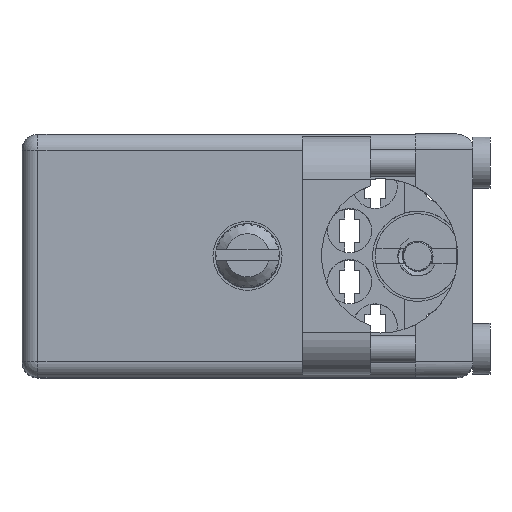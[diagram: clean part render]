
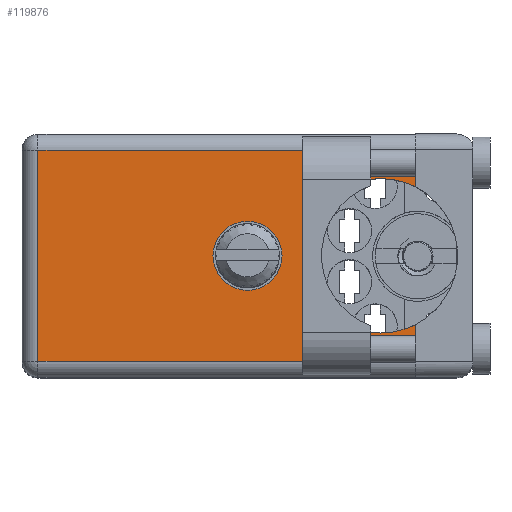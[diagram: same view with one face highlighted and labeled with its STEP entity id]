
A CAD part, top view. The second image highlights one B-rep face of the part: STEP entity #119876.
In plain terms, the highlighted face is planar.
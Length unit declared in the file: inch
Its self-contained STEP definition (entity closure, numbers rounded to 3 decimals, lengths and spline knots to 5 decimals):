
#12 = ORIENTED_EDGE ( 'NONE', *, *, #181974, .F. ) ;
#953 = EDGE_LOOP ( 'NONE', ( #184170, #178870, #45700, #61949, #62573, #991, #3942, #164983 ) ) ;
#991 = ORIENTED_EDGE ( 'NONE', *, *, #170687, .F. ) ;
#3942 = ORIENTED_EDGE ( 'NONE', *, *, #40026, .F. ) ;
#6084 = LINE ( 'NONE', #177541, #95684 ) ;
#7686 = CARTESIAN_POINT ( 'NONE',  ( 1.155, 0.906, -0.047 ) ) ;
#15477 = VERTEX_POINT ( 'NONE', #7686 ) ;
#15964 = EDGE_CURVE ( 'NONE', #175956, #15477, #23277, .T. ) ;
#17097 = EDGE_CURVE ( 'NONE', #26649, #60607, #51531, .T. ) ;
#17953 = DIRECTION ( 'NONE',  ( 0., 0., 1. ) ) ;
#20714 = AXIS2_PLACEMENT_3D ( 'NONE', #136586, #75239, #121382 ) ;
#21049 = CARTESIAN_POINT ( 'NONE',  ( 1.155, 0.906, -0.15471 ) ) ;
#22988 = CARTESIAN_POINT ( 'NONE',  ( 0.6625, 0.906, -0.3575 ) ) ;
#23277 = LINE ( 'NONE', #110480, #178972 ) ;
#26649 = VERTEX_POINT ( 'NONE', #158919 ) ;
#26757 = CARTESIAN_POINT ( 'NONE',  ( 1.155, 0.906, 0. ) ) ;
#27694 = DIRECTION ( 'NONE',  ( 0., 1., 0. ) ) ;
#28129 = CARTESIAN_POINT ( 'NONE',  ( 0.047, 0.906, -0.047 ) ) ;
#31699 = AXIS2_PLACEMENT_3D ( 'NONE', #116011, #189311, #38981 ) ;
#33539 = ORIENTED_EDGE ( 'NONE', *, *, #17097, .F. ) ;
#37393 = DIRECTION ( 'NONE',  ( 0., 1., 0. ) ) ;
#38981 = DIRECTION ( 'NONE',  ( 0., 0., 1. ) ) ;
#39547 = CIRCLE ( 'NONE', #159974, 0.227 ) ;
#39955 = DIRECTION ( 'NONE',  ( 0., 0., 1. ) ) ;
#40026 = EDGE_CURVE ( 'NONE', #125708, #55909, #39547, .T. ) ;
#45034 = VERTEX_POINT ( 'NONE', #101981 ) ;
#45109 = FACE_OUTER_BOUND ( 'NONE', #953, .T. ) ;
#45700 = ORIENTED_EDGE ( 'NONE', *, *, #111806, .T. ) ;
#51531 = CIRCLE ( 'NONE', #166721, 0.1015 ) ;
#55909 = VERTEX_POINT ( 'NONE', #116212 ) ;
#60607 = VERTEX_POINT ( 'NONE', #114581 ) ;
#61949 = ORIENTED_EDGE ( 'NONE', *, *, #15964, .T. ) ;
#62573 = ORIENTED_EDGE ( 'NONE', *, *, #193904, .F. ) ;
#62931 = VERTEX_POINT ( 'NONE', #87518 ) ;
#65061 = DIRECTION ( 'NONE',  ( 1., 0., 0. ) ) ;
#71324 = CARTESIAN_POINT ( 'NONE',  ( 1.155, 0.906, 0. ) ) ;
#72088 = DIRECTION ( 'NONE',  ( -1., 0., 0. ) ) ;
#75239 = DIRECTION ( 'NONE',  ( 0., 1., 0. ) ) ;
#83783 = EDGE_CURVE ( 'NONE', #62931, #188450, #99415, .T. ) ;
#84217 = DIRECTION ( 'NONE',  ( 0., 0., 1. ) ) ;
#87134 = DIRECTION ( 'NONE',  ( 0., 0., 1. ) ) ;
#87518 = CARTESIAN_POINT ( 'NONE',  ( 1.155, 0.906, -0.668 ) ) ;
#89527 = VERTEX_POINT ( 'NONE', #21049 ) ;
#89919 = VECTOR ( 'NONE', #39955, 39.37008 ) ;
#92616 = VECTOR ( 'NONE', #87134, 39.37008 ) ;
#95684 = VECTOR ( 'NONE', #178829, 39.37008 ) ;
#99415 = LINE ( 'NONE', #26757, #89919 ) ;
#101642 = EDGE_CURVE ( 'NONE', #188450, #125708, #107735, .T. ) ;
#101981 = CARTESIAN_POINT ( 'NONE',  ( 0.047, 0.906, -0.668 ) ) ;
#107735 = CIRCLE ( 'NONE', #31699, 0.227 ) ;
#110480 = CARTESIAN_POINT ( 'NONE',  ( 1.155, 0.906, -0.047 ) ) ;
#111565 = VECTOR ( 'NONE', #72088, 39.37008 ) ;
#111806 = EDGE_CURVE ( 'NONE', #45034, #175956, #6084, .T. ) ;
#113498 = FACE_BOUND ( 'NONE', #128687, .T. ) ;
#114581 = CARTESIAN_POINT ( 'NONE',  ( 0.6625, 0.906, -0.459 ) ) ;
#115311 = DIRECTION ( 'NONE',  ( 0., 0., 1. ) ) ;
#116011 = CARTESIAN_POINT ( 'NONE',  ( 1.053, 0.906, -0.3575 ) ) ;
#116212 = CARTESIAN_POINT ( 'NONE',  ( 1.053, 0.906, -0.1305 ) ) ;
#116341 = LINE ( 'NONE', #118855, #111565 ) ;
#118855 = CARTESIAN_POINT ( 'NONE',  ( 0., 0.906, -0.668 ) ) ;
#119876 = ADVANCED_FACE ( 'NONE', ( #45109, #113498 ), #165583, .T. ) ;
#121382 = DIRECTION ( 'NONE',  ( 0., 0., 1. ) ) ;
#123709 = AXIS2_PLACEMENT_3D ( 'NONE', #22988, #128479, #84217 ) ;
#125708 = VERTEX_POINT ( 'NONE', #181642 ) ;
#127070 = DIRECTION ( 'NONE',  ( 0., 0., 1. ) ) ;
#128479 = DIRECTION ( 'NONE',  ( 0., 1., 0. ) ) ;
#128687 = EDGE_LOOP ( 'NONE', ( #33539, #12 ) ) ;
#130353 = EDGE_CURVE ( 'NONE', #62931, #45034, #116341, .T. ) ;
#130623 = AXIS2_PLACEMENT_3D ( 'NONE', #193172, #27694, #115311 ) ;
#136586 = CARTESIAN_POINT ( 'NONE',  ( 0., 0.906, -0.715 ) ) ;
#136610 = DIRECTION ( 'NONE',  ( 0., 1., 0. ) ) ;
#141553 = CARTESIAN_POINT ( 'NONE',  ( 0.6625, 0.906, -0.3575 ) ) ;
#156234 = CARTESIAN_POINT ( 'NONE',  ( 1.155, 0.906, -0.56029 ) ) ;
#158919 = CARTESIAN_POINT ( 'NONE',  ( 0.6625, 0.906, -0.256 ) ) ;
#159974 = AXIS2_PLACEMENT_3D ( 'NONE', #168223, #136610, #17953 ) ;
#164983 = ORIENTED_EDGE ( 'NONE', *, *, #101642, .F. ) ;
#165583 = PLANE ( 'NONE',  #20714 ) ;
#165918 = LINE ( 'NONE', #71324, #92616 ) ;
#166721 = AXIS2_PLACEMENT_3D ( 'NONE', #141553, #37393, #127070 ) ;
#168223 = CARTESIAN_POINT ( 'NONE',  ( 1.053, 0.906, -0.3575 ) ) ;
#170687 = EDGE_CURVE ( 'NONE', #55909, #89527, #173046, .T. ) ;
#173046 = CIRCLE ( 'NONE', #130623, 0.227 ) ;
#175956 = VERTEX_POINT ( 'NONE', #28129 ) ;
#177541 = CARTESIAN_POINT ( 'NONE',  ( 0.047, 0.906, -0.715 ) ) ;
#178829 = DIRECTION ( 'NONE',  ( 0., 0., 1. ) ) ;
#178870 = ORIENTED_EDGE ( 'NONE', *, *, #130353, .T. ) ;
#178972 = VECTOR ( 'NONE', #65061, 39.37008 ) ;
#181642 = CARTESIAN_POINT ( 'NONE',  ( 1.053, 0.906, -0.5845 ) ) ;
#181974 = EDGE_CURVE ( 'NONE', #60607, #26649, #187931, .T. ) ;
#184170 = ORIENTED_EDGE ( 'NONE', *, *, #83783, .F. ) ;
#187931 = CIRCLE ( 'NONE', #123709, 0.1015 ) ;
#188450 = VERTEX_POINT ( 'NONE', #156234 ) ;
#189311 = DIRECTION ( 'NONE',  ( 0., 1., 0. ) ) ;
#193172 = CARTESIAN_POINT ( 'NONE',  ( 1.053, 0.906, -0.3575 ) ) ;
#193904 = EDGE_CURVE ( 'NONE', #89527, #15477, #165918, .T. ) ;
